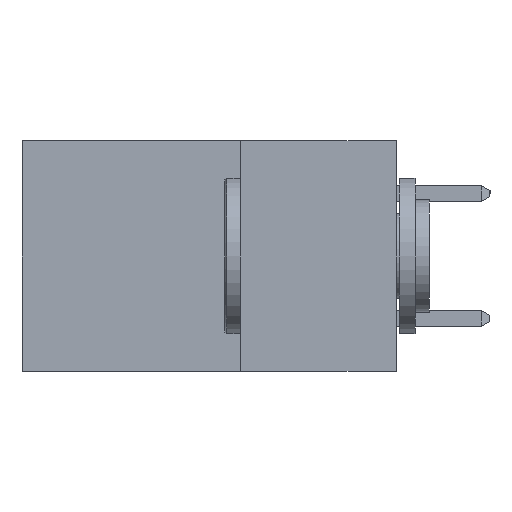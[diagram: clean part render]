
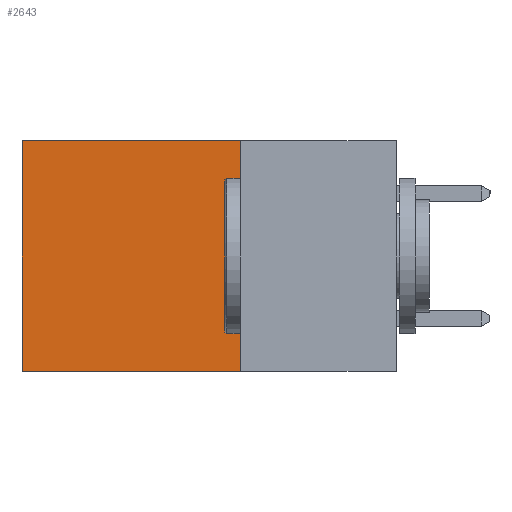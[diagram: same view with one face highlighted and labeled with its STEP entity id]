
A CAD part, left-side view. The second image highlights one B-rep face of the part: STEP entity #2643.
In plain terms, the highlighted planar face has unit normal (-1, 0, 0).
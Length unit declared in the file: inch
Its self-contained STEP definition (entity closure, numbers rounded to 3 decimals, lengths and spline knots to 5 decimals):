
#1648 = EDGE_LOOP ( 'NONE', ( #14136, #15514, #3969, #7956 ) ) ;
#1918 = DIRECTION ( 'NONE',  ( 0., 0., -1. ) ) ;
#1927 = DIRECTION ( 'NONE',  ( 0., 0., -1. ) ) ;
#1989 = DIRECTION ( 'NONE',  ( 0., 1., 0. ) ) ;
#2579 = LINE ( 'NONE', #12386, #13544 ) ;
#2643 = ADVANCED_FACE ( 'NONE', ( #15347 ), #12803, .F. ) ;
#3213 = VERTEX_POINT ( 'NONE', #6578 ) ;
#3315 = DIRECTION ( 'NONE',  ( 0., 0., -1. ) ) ;
#3589 = VECTOR ( 'NONE', #3315, 39.37008 ) ;
#3969 = ORIENTED_EDGE ( 'NONE', *, *, #4010, .F. ) ;
#4010 = EDGE_CURVE ( 'NONE', #13221, #3213, #15216, .T. ) ;
#5581 = VECTOR ( 'NONE', #1989, 39.37008 ) ;
#5616 = LINE ( 'NONE', #14005, #13636 ) ;
#6125 = CARTESIAN_POINT ( 'NONE',  ( 0.2615, 0.25, -0.37 ) ) ;
#6256 = CARTESIAN_POINT ( 'NONE',  ( 0.2615, 0.25, -0.37 ) ) ;
#6578 = CARTESIAN_POINT ( 'NONE',  ( 0.2615, 0.25, -0.37 ) ) ;
#6713 = EDGE_CURVE ( 'NONE', #8019, #11788, #5616, .T. ) ;
#7234 = EDGE_CURVE ( 'NONE', #3213, #11788, #9071, .T. ) ;
#7956 = ORIENTED_EDGE ( 'NONE', *, *, #14725, .T. ) ;
#8019 = VERTEX_POINT ( 'NONE', #9789 ) ;
#9071 = LINE ( 'NONE', #10038, #5581 ) ;
#9234 = AXIS2_PLACEMENT_3D ( 'NONE', #6256, #11666, #1927 ) ;
#9789 = CARTESIAN_POINT ( 'NONE',  ( 0.2615, 0.6, 0. ) ) ;
#10038 = CARTESIAN_POINT ( 'NONE',  ( 0.2615, 0.25, -0.37 ) ) ;
#11666 = DIRECTION ( 'NONE',  ( 1., 0., 0. ) ) ;
#11788 = VERTEX_POINT ( 'NONE', #12833 ) ;
#12300 = DIRECTION ( 'NONE',  ( 0., 1., 0. ) ) ;
#12386 = CARTESIAN_POINT ( 'NONE',  ( 0.2615, 0.25, 0. ) ) ;
#12803 = PLANE ( 'NONE',  #9234 ) ;
#12833 = CARTESIAN_POINT ( 'NONE',  ( 0.2615, 0.6, -0.37 ) ) ;
#13221 = VERTEX_POINT ( 'NONE', #16141 ) ;
#13544 = VECTOR ( 'NONE', #12300, 39.37008 ) ;
#13636 = VECTOR ( 'NONE', #1918, 39.37008 ) ;
#14005 = CARTESIAN_POINT ( 'NONE',  ( 0.2615, 0.6, -0.37 ) ) ;
#14136 = ORIENTED_EDGE ( 'NONE', *, *, #6713, .T. ) ;
#14725 = EDGE_CURVE ( 'NONE', #13221, #8019, #2579, .T. ) ;
#15216 = LINE ( 'NONE', #6125, #3589 ) ;
#15347 = FACE_OUTER_BOUND ( 'NONE', #1648, .T. ) ;
#15514 = ORIENTED_EDGE ( 'NONE', *, *, #7234, .F. ) ;
#16141 = CARTESIAN_POINT ( 'NONE',  ( 0.2615, 0.25, 0. ) ) ;
